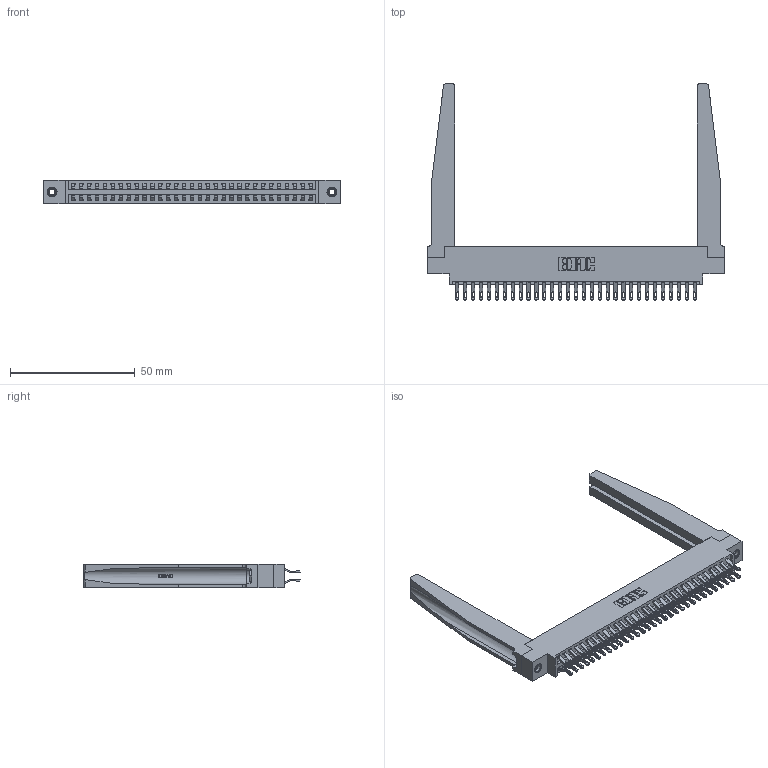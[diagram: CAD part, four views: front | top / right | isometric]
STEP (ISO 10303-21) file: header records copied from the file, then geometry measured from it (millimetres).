
FILE_DESCRIPTION (( 'STEP AP203' ), '1' );
FILE_NAME ('396-062-555-878.STEP', '2019-11-02T09:28:36', ( '' ), ( '' ), 'SwSTEP 2.0', 'SolidWorks 2016', '' );
FILE_SCHEMA (( 'CONFIG_CONTROL_DESIGN' ));
Length unit declared in the file: inch
Products named in the file (5): 346 Part_0.170 Offset - 0.156 Dia-TH; 345-292-001_555 Tail; 346-220-078_345-220-078; 396-062-555-878; 345-250-001_345-250-001-102
Assembly tree (67 placements, depth 2):
  396-062-555-878
    346 Part_0.170 Offset - 0.156 Dia-TH
    345-292-001_555 Tail  x62
    346-220-078_345-220-078  x2
    345-250-001_345-250-001-102  x2
Bounding box: 119 x 86.74 x 9.4 mm (x, y, z)
Volume: 18452.5 mm3; surface area: 23052.8 mm2
Topology: 67 solids, 67 shells, 3956 faces, 12295 edges, 8186 vertices
Faces by surface type: plane 2268, cylinder 1636, bspline 36, cone 12, torus 4
Entity records: 26918 total; most frequent: CARTESIAN_POINT 5425, ORIENTED_EDGE 4218, DIRECTION 3787, EDGE_CURVE 2109, LINE 1739, VECTOR 1739, VERTEX_POINT 1400, AXIS2_PLACEMENT_3D 1024
